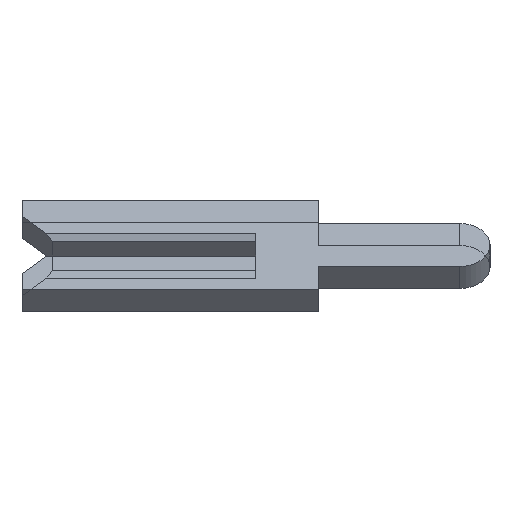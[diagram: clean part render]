
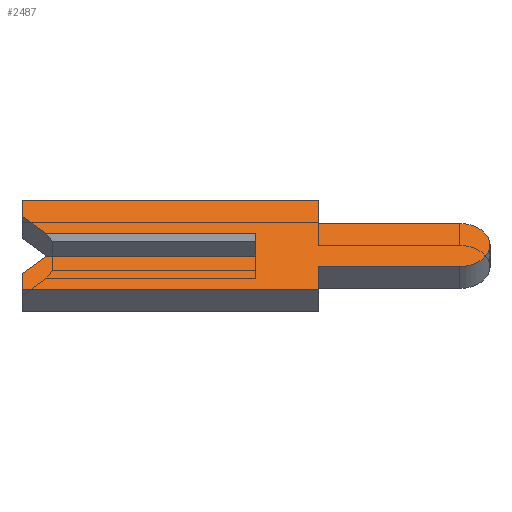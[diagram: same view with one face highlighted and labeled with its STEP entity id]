
A CAD part, left-side view. The second image highlights one B-rep face of the part: STEP entity #2487.
In plain terms, the highlighted face is planar.
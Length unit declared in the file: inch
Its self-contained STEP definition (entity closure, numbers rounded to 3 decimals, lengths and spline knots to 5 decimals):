
#28 = LINE ( 'NONE', #120, #989 ) ;
#32 = ORIENTED_EDGE ( 'NONE', *, *, #2360, .F. ) ;
#47 = ORIENTED_EDGE ( 'NONE', *, *, #886, .F. ) ;
#120 = CARTESIAN_POINT ( 'NONE',  ( -0.01, 0.15, -0.04 ) ) ;
#182 = ORIENTED_EDGE ( 'NONE', *, *, #2395, .F. ) ;
#203 = LINE ( 'NONE', #1614, #3455 ) ;
#237 = CARTESIAN_POINT ( 'NONE',  ( -0.01, 0.15, 0.04 ) ) ;
#245 = LINE ( 'NONE', #952, #1584 ) ;
#255 = ORIENTED_EDGE ( 'NONE', *, *, #2565, .F. ) ;
#284 = DIRECTION ( 'NONE',  ( 0., 0., -1. ) ) ;
#328 = CARTESIAN_POINT ( 'NONE',  ( -0.01, 0.15, 0.026 ) ) ;
#345 = ORIENTED_EDGE ( 'NONE', *, *, #1375, .F. ) ;
#444 = VECTOR ( 'NONE', #1460, 39.37008 ) ;
#617 = CARTESIAN_POINT ( 'NONE',  ( -0.01, -0.1305, 0. ) ) ;
#630 = CARTESIAN_POINT ( 'NONE',  ( -0.01, -0.04, -0.04 ) ) ;
#668 = CARTESIAN_POINT ( 'NONE',  ( -0.01, 0.15, 0.026 ) ) ;
#746 = VECTOR ( 'NONE', #1893, 39.37008 ) ;
#761 = EDGE_LOOP ( 'NONE', ( #1199, #345, #1568, #834, #1339, #47, #32, #255, #2919, #3910, #182, #3115, #2799, #1878 ) ) ;
#791 = VERTEX_POINT ( 'NONE', #2992 ) ;
#797 = VECTOR ( 'NONE', #885, 39.37008 ) ;
#808 = EDGE_CURVE ( 'NONE', #791, #1078, #1629, .T. ) ;
#834 = ORIENTED_EDGE ( 'NONE', *, *, #1803, .F. ) ;
#885 = DIRECTION ( 'NONE',  ( 0., 0., 1. ) ) ;
#886 = EDGE_CURVE ( 'NONE', #2622, #1084, #28, .T. ) ;
#952 = CARTESIAN_POINT ( 'NONE',  ( -0.01, -0.1305, -0.01 ) ) ;
#989 = VECTOR ( 'NONE', #1089, 39.37008 ) ;
#1003 = VERTEX_POINT ( 'NONE', #3071 ) ;
#1043 = VECTOR ( 'NONE', #284, 39.37008 ) ;
#1078 = VERTEX_POINT ( 'NONE', #1479 ) ;
#1084 = VERTEX_POINT ( 'NONE', #1166 ) ;
#1089 = DIRECTION ( 'NONE',  ( 0., 1., 0. ) ) ;
#1108 = VERTEX_POINT ( 'NONE', #237 ) ;
#1166 = CARTESIAN_POINT ( 'NONE',  ( -0.01, 0.15, -0.04 ) ) ;
#1199 = ORIENTED_EDGE ( 'NONE', *, *, #808, .T. ) ;
#1212 = CARTESIAN_POINT ( 'NONE',  ( -0.01, -0.1305, -0.0195 ) ) ;
#1222 = EDGE_CURVE ( 'NONE', #1084, #2575, #1727, .T. ) ;
#1251 = DIRECTION ( 'NONE',  ( 0., -1., 0. ) ) ;
#1339 = ORIENTED_EDGE ( 'NONE', *, *, #1222, .F. ) ;
#1375 = EDGE_CURVE ( 'NONE', #1593, #1078, #2686, .T. ) ;
#1406 = EDGE_CURVE ( 'NONE', #791, #2879, #2865, .T. ) ;
#1460 = DIRECTION ( 'NONE',  ( 0., 0.707, 0.707 ) ) ;
#1479 = CARTESIAN_POINT ( 'NONE',  ( -0.01, 0., 0.01 ) ) ;
#1517 = PLANE ( 'NONE',  #3124 ) ;
#1526 = VERTEX_POINT ( 'NONE', #2726 ) ;
#1568 = ORIENTED_EDGE ( 'NONE', *, *, #2446, .F. ) ;
#1584 = VECTOR ( 'NONE', #1251, 39.37008 ) ;
#1593 = VERTEX_POINT ( 'NONE', #2086 ) ;
#1614 = CARTESIAN_POINT ( 'NONE',  ( -0.01, -0.04, 0.0195 ) ) ;
#1626 = DIRECTION ( 'NONE',  ( 0., 0., -1. ) ) ;
#1629 = LINE ( 'NONE', #2375, #3200 ) ;
#1727 = LINE ( 'NONE', #2112, #797 ) ;
#1778 = CARTESIAN_POINT ( 'NONE',  ( -0.01, 0.1305, 0.0065 ) ) ;
#1781 = LINE ( 'NONE', #3239, #2325 ) ;
#1803 = EDGE_CURVE ( 'NONE', #2575, #2416, #2028, .T. ) ;
#1831 = CARTESIAN_POINT ( 'NONE',  ( -0.01, -0.04, -0.0195 ) ) ;
#1877 = LINE ( 'NONE', #2790, #1043 ) ;
#1878 = ORIENTED_EDGE ( 'NONE', *, *, #1406, .F. ) ;
#1893 = DIRECTION ( 'NONE',  ( 0., 1., 0. ) ) ;
#1904 = DIRECTION ( 'NONE',  ( 0., 0., 1. ) ) ;
#1949 = DIRECTION ( 'NONE',  ( 0., -1., 0. ) ) ;
#2028 = LINE ( 'NONE', #2101, #3749 ) ;
#2086 = CARTESIAN_POINT ( 'NONE',  ( -0.01, 0., -0.01 ) ) ;
#2101 = CARTESIAN_POINT ( 'NONE',  ( -0.01, 0.1305, -0.0065 ) ) ;
#2112 = CARTESIAN_POINT ( 'NONE',  ( -0.01, 0.15, -0.026 ) ) ;
#2129 = CARTESIAN_POINT ( 'NONE',  ( -0.01, 0., 0.0065 ) ) ;
#2137 = LINE ( 'NONE', #1831, #746 ) ;
#2146 = EDGE_CURVE ( 'NONE', #1526, #2525, #2815, .T. ) ;
#2245 = CARTESIAN_POINT ( 'NONE',  ( -0.01, 0.15, -0.026 ) ) ;
#2296 = DIRECTION ( 'NONE',  ( 0., -1., 0. ) ) ;
#2325 = VECTOR ( 'NONE', #2296, 39.37008 ) ;
#2360 = EDGE_CURVE ( 'NONE', #3960, #2622, #2435, .T. ) ;
#2375 = CARTESIAN_POINT ( 'NONE',  ( -0.01, 0.15, 0.01 ) ) ;
#2395 = EDGE_CURVE ( 'NONE', #3730, #1003, #1877, .T. ) ;
#2416 = VERTEX_POINT ( 'NONE', #3741 ) ;
#2435 = LINE ( 'NONE', #630, #3659 ) ;
#2446 = EDGE_CURVE ( 'NONE', #2416, #1593, #245, .T. ) ;
#2487 = ADVANCED_FACE ( 'NONE', ( #3800 ), #1517, .F. ) ;
#2525 = VERTEX_POINT ( 'NONE', #1212 ) ;
#2565 = EDGE_CURVE ( 'NONE', #2525, #3960, #2137, .T. ) ;
#2575 = VERTEX_POINT ( 'NONE', #2245 ) ;
#2604 = CARTESIAN_POINT ( 'NONE',  ( -0.01, -0.04, -0.0195 ) ) ;
#2622 = VERTEX_POINT ( 'NONE', #2780 ) ;
#2686 = LINE ( 'NONE', #2129, #3475 ) ;
#2726 = CARTESIAN_POINT ( 'NONE',  ( -0.01, -0.1305, 0.0195 ) ) ;
#2768 = DIRECTION ( 'NONE',  ( 0., 0., 1. ) ) ;
#2780 = CARTESIAN_POINT ( 'NONE',  ( -0.01, -0.04, -0.04 ) ) ;
#2782 = EDGE_CURVE ( 'NONE', #2879, #1108, #3255, .T. ) ;
#2790 = CARTESIAN_POINT ( 'NONE',  ( -0.01, -0.04, 0.04 ) ) ;
#2799 = ORIENTED_EDGE ( 'NONE', *, *, #2782, .F. ) ;
#2815 = CIRCLE ( 'NONE', #3056, 0.0195 ) ;
#2821 = DIRECTION ( 'NONE',  ( 0., 0., -1. ) ) ;
#2832 = DIRECTION ( 'NONE',  ( 0., 0., -1. ) ) ;
#2865 = LINE ( 'NONE', #1778, #444 ) ;
#2870 = CARTESIAN_POINT ( 'NONE',  ( -0.01, -0.1305, 0. ) ) ;
#2879 = VERTEX_POINT ( 'NONE', #328 ) ;
#2919 = ORIENTED_EDGE ( 'NONE', *, *, #2146, .F. ) ;
#2992 = CARTESIAN_POINT ( 'NONE',  ( -0.01, 0.134, 0.01 ) ) ;
#3056 = AXIS2_PLACEMENT_3D ( 'NONE', #2870, #3500, #1626 ) ;
#3071 = CARTESIAN_POINT ( 'NONE',  ( -0.01, -0.04, 0.0195 ) ) ;
#3072 = EDGE_CURVE ( 'NONE', #1003, #1526, #203, .T. ) ;
#3108 = DIRECTION ( 'NONE',  ( 1., 0., 0. ) ) ;
#3115 = ORIENTED_EDGE ( 'NONE', *, *, #3705, .F. ) ;
#3124 = AXIS2_PLACEMENT_3D ( 'NONE', #617, #3108, #2821 ) ;
#3200 = VECTOR ( 'NONE', #3274, 39.37008 ) ;
#3239 = CARTESIAN_POINT ( 'NONE',  ( -0.01, 0.15, 0.04 ) ) ;
#3255 = LINE ( 'NONE', #668, #3688 ) ;
#3274 = DIRECTION ( 'NONE',  ( 0., -1., 0. ) ) ;
#3414 = DIRECTION ( 'NONE',  ( 0., -0.707, 0.707 ) ) ;
#3455 = VECTOR ( 'NONE', #1949, 39.37008 ) ;
#3475 = VECTOR ( 'NONE', #2768, 39.37008 ) ;
#3500 = DIRECTION ( 'NONE',  ( 1., 0., 0. ) ) ;
#3555 = CARTESIAN_POINT ( 'NONE',  ( -0.01, -0.04, 0.04 ) ) ;
#3659 = VECTOR ( 'NONE', #2832, 39.37008 ) ;
#3688 = VECTOR ( 'NONE', #1904, 39.37008 ) ;
#3705 = EDGE_CURVE ( 'NONE', #1108, #3730, #1781, .T. ) ;
#3730 = VERTEX_POINT ( 'NONE', #3555 ) ;
#3741 = CARTESIAN_POINT ( 'NONE',  ( -0.01, 0.134, -0.01 ) ) ;
#3749 = VECTOR ( 'NONE', #3414, 39.37008 ) ;
#3800 = FACE_OUTER_BOUND ( 'NONE', #761, .T. ) ;
#3910 = ORIENTED_EDGE ( 'NONE', *, *, #3072, .F. ) ;
#3960 = VERTEX_POINT ( 'NONE', #2604 ) ;
